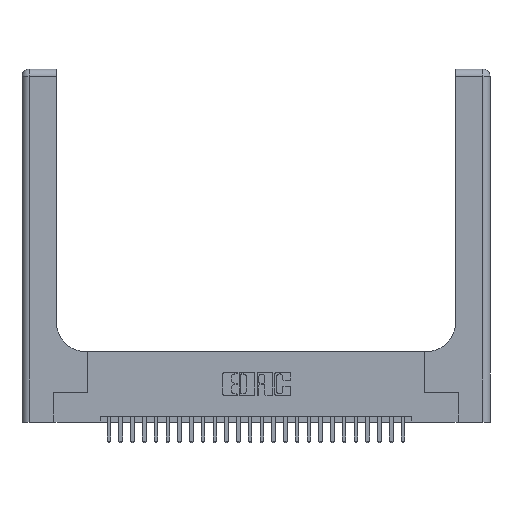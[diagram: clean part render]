
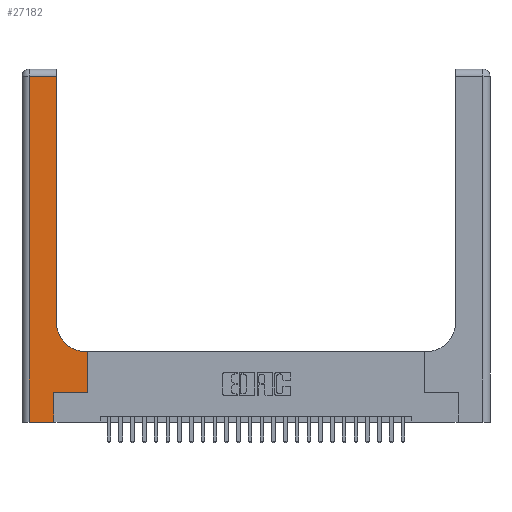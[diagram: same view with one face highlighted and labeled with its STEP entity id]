
A CAD part, top view. The second image highlights one B-rep face of the part: STEP entity #27182.
In plain terms, the highlighted planar face has unit normal (0, 0, 1).
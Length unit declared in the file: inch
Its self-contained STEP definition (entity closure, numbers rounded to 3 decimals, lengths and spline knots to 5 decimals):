
#211 = DIRECTION ( 'NONE',  ( -1., 0., 0. ) ) ;
#458 = CARTESIAN_POINT ( 'NONE',  ( 0.269, 0.25, 0.37 ) ) ;
#740 = CARTESIAN_POINT ( 'NONE',  ( 0.5415, 0.6, 0.37 ) ) ;
#850 = ORIENTED_EDGE ( 'NONE', *, *, #5907, .T. ) ;
#990 = VERTEX_POINT ( 'NONE', #25654 ) ;
#1175 = DIRECTION ( 'NONE',  ( 1., 0., 0. ) ) ;
#2775 = VECTOR ( 'NONE', #7517, 39.37008 ) ;
#3098 = CARTESIAN_POINT ( 'NONE',  ( 0.5585, 0.25, 0.37 ) ) ;
#3229 = ORIENTED_EDGE ( 'NONE', *, *, #13736, .T. ) ;
#4087 = DIRECTION ( 'NONE',  ( 0., 1., 0. ) ) ;
#4631 = CARTESIAN_POINT ( 'NONE',  ( 0., 0., 0.37 ) ) ;
#4775 = EDGE_CURVE ( 'NONE', #5201, #5668, #17483, .T. ) ;
#4805 = LINE ( 'NONE', #6473, #26979 ) ;
#4828 = EDGE_CURVE ( 'NONE', #11036, #18460, #16104, .T. ) ;
#5201 = VERTEX_POINT ( 'NONE', #8184 ) ;
#5668 = VERTEX_POINT ( 'NONE', #22519 ) ;
#5752 = AXIS2_PLACEMENT_3D ( 'NONE', #9256, #24274, #11436 ) ;
#5907 = EDGE_CURVE ( 'NONE', #18460, #21161, #17057, .T. ) ;
#6015 = ORIENTED_EDGE ( 'NONE', *, *, #4775, .T. ) ;
#6165 = EDGE_CURVE ( 'NONE', #12696, #21416, #11672, .T. ) ;
#6473 = CARTESIAN_POINT ( 'NONE',  ( 0.2915, 3., 0.37 ) ) ;
#7517 = DIRECTION ( 'NONE',  ( 0., 1., 0. ) ) ;
#8110 = ORIENTED_EDGE ( 'NONE', *, *, #9634, .T. ) ;
#8184 = CARTESIAN_POINT ( 'NONE',  ( 0.06, 0., 0.37 ) ) ;
#8386 = FACE_OUTER_BOUND ( 'NONE', #18929, .T. ) ;
#8609 = DIRECTION ( 'NONE',  ( 0., -1., 0. ) ) ;
#8812 = PLANE ( 'NONE',  #20060 ) ;
#9256 = CARTESIAN_POINT ( 'NONE',  ( 0.5415, 0.85, 0.37 ) ) ;
#9634 = EDGE_CURVE ( 'NONE', #21161, #12696, #17553, .T. ) ;
#10352 = VERTEX_POINT ( 'NONE', #12452 ) ;
#10399 = VECTOR ( 'NONE', #21994, 39.37008 ) ;
#10529 = CARTESIAN_POINT ( 'NONE',  ( 0., 2.94, 0.37 ) ) ;
#10804 = LINE ( 'NONE', #23626, #27263 ) ;
#11036 = VERTEX_POINT ( 'NONE', #23770 ) ;
#11362 = VECTOR ( 'NONE', #4087, 39.37008 ) ;
#11436 = DIRECTION ( 'NONE',  ( 1., 0., 0. ) ) ;
#11672 = CIRCLE ( 'NONE', #5752, 0.25 ) ;
#12293 = CARTESIAN_POINT ( 'NONE',  ( 0.2915, 0.6, 0.37 ) ) ;
#12452 = CARTESIAN_POINT ( 'NONE',  ( 0.2915, 2.94, 0.37 ) ) ;
#12696 = VERTEX_POINT ( 'NONE', #740 ) ;
#13142 = DIRECTION ( 'NONE',  ( 0., 0., -1. ) ) ;
#13715 = ORIENTED_EDGE ( 'NONE', *, *, #19134, .T. ) ;
#13736 = EDGE_CURVE ( 'NONE', #990, #5201, #10804, .T. ) ;
#15679 = LINE ( 'NONE', #10529, #25071 ) ;
#15807 = ORIENTED_EDGE ( 'NONE', *, *, #4828, .T. ) ;
#16104 = LINE ( 'NONE', #458, #10399 ) ;
#16546 = EDGE_CURVE ( 'NONE', #10352, #990, #15679, .T. ) ;
#16651 = CARTESIAN_POINT ( 'NONE',  ( 0.5585, 0.6, 0.37 ) ) ;
#17057 = LINE ( 'NONE', #21276, #11362 ) ;
#17483 = LINE ( 'NONE', #4631, #23846 ) ;
#17553 = LINE ( 'NONE', #12293, #18209 ) ;
#18209 = VECTOR ( 'NONE', #25142, 39.37008 ) ;
#18247 = ORIENTED_EDGE ( 'NONE', *, *, #16546, .T. ) ;
#18460 = VERTEX_POINT ( 'NONE', #3098 ) ;
#18929 = EDGE_LOOP ( 'NONE', ( #20405, #18247, #3229, #6015, #13715, #15807, #850, #8110, #21959 ) ) ;
#19134 = EDGE_CURVE ( 'NONE', #5668, #11036, #24966, .T. ) ;
#19197 = DIRECTION ( 'NONE',  ( -1., 0., 0. ) ) ;
#20060 = AXIS2_PLACEMENT_3D ( 'NONE', #25976, #13142, #211 ) ;
#20394 = CARTESIAN_POINT ( 'NONE',  ( 0.269, 0., 0.37 ) ) ;
#20405 = ORIENTED_EDGE ( 'NONE', *, *, #24757, .T. ) ;
#21161 = VERTEX_POINT ( 'NONE', #16651 ) ;
#21276 = CARTESIAN_POINT ( 'NONE',  ( 0.5585, 0.25, 0.37 ) ) ;
#21416 = VERTEX_POINT ( 'NONE', #26029 ) ;
#21959 = ORIENTED_EDGE ( 'NONE', *, *, #6165, .T. ) ;
#21994 = DIRECTION ( 'NONE',  ( 1., 0., 0. ) ) ;
#22519 = CARTESIAN_POINT ( 'NONE',  ( 0.269, 0., 0.37 ) ) ;
#23626 = CARTESIAN_POINT ( 'NONE',  ( 0.06, 3., 0.37 ) ) ;
#23770 = CARTESIAN_POINT ( 'NONE',  ( 0.269, 0.25, 0.37 ) ) ;
#23846 = VECTOR ( 'NONE', #1175, 39.37008 ) ;
#24274 = DIRECTION ( 'NONE',  ( 0., 0., -1. ) ) ;
#24757 = EDGE_CURVE ( 'NONE', #21416, #10352, #4805, .T. ) ;
#24966 = LINE ( 'NONE', #20394, #2775 ) ;
#25071 = VECTOR ( 'NONE', #19197, 39.37008 ) ;
#25142 = DIRECTION ( 'NONE',  ( -1., 0., 0. ) ) ;
#25654 = CARTESIAN_POINT ( 'NONE',  ( 0.06, 2.94, 0.37 ) ) ;
#25734 = DIRECTION ( 'NONE',  ( 0., 1., 0. ) ) ;
#25976 = CARTESIAN_POINT ( 'NONE',  ( 0., 3., 0.37 ) ) ;
#26029 = CARTESIAN_POINT ( 'NONE',  ( 0.2915, 0.85, 0.37 ) ) ;
#26979 = VECTOR ( 'NONE', #25734, 39.37008 ) ;
#27182 = ADVANCED_FACE ( 'NONE', ( #8386 ), #8812, .F. ) ;
#27263 = VECTOR ( 'NONE', #8609, 39.37008 ) ;
